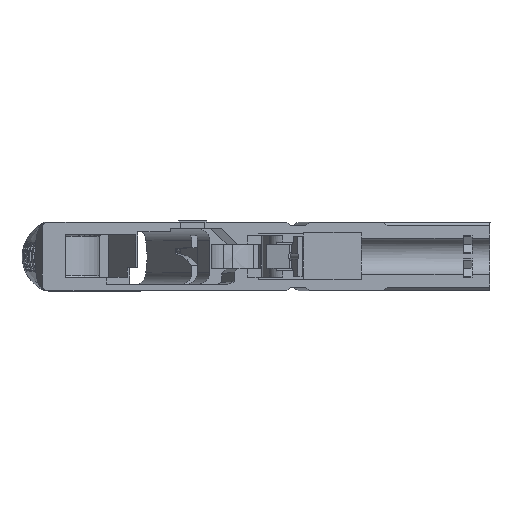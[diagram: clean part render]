
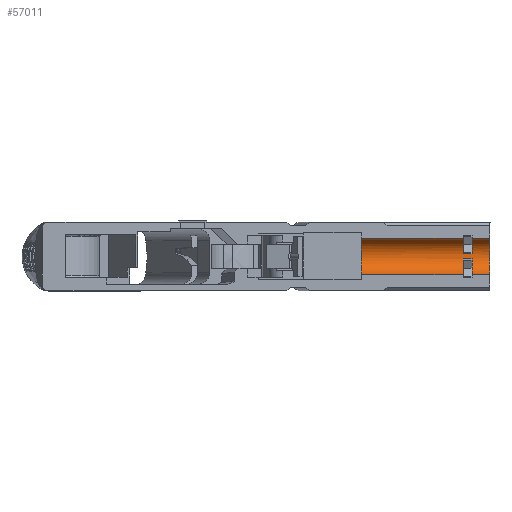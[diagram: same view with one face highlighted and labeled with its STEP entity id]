
A CAD part, top view. The second image highlights one B-rep face of the part: STEP entity #57011.
In plain terms, the highlighted cylindrical face has radius 7.768 mm (diameter 15.535 mm), a partial arc.
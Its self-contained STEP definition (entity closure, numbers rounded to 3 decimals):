
#6073=CYLINDRICAL_SURFACE('',#60469,7.768);
#7816=CIRCLE('',#60417,7.768);
#7819=CIRCLE('',#60444,7.768);
#7824=CIRCLE('',#60450,7.768);
#7827=CIRCLE('',#60465,7.768);
#7828=CIRCLE('',#60467,7.768);
#7829=CIRCLE('',#60470,7.768);
#8081=FACE_OUTER_BOUND('',#11523,.T.);
#11523=EDGE_LOOP('',(#38179,#38180,#38181,#38182,#38183,#38184,#38185,#38186,
#38187,#38188,#38189,#38190,#38191,#38192));
#15564=LINE('',#68849,#19314);
#15572=LINE('',#68868,#19322);
#15574=LINE('',#68871,#19324);
#15575=LINE('',#68873,#19325);
#15576=LINE('',#68876,#19326);
#15577=LINE('',#68877,#19327);
#15578=LINE('',#68879,#19328);
#15579=LINE('',#68880,#19329);
#19314=VECTOR('',#62119,10.);
#19322=VECTOR('',#62139,10.);
#19324=VECTOR('',#62143,10.);
#19325=VECTOR('',#62144,10.);
#19326=VECTOR('',#62147,10.);
#19327=VECTOR('',#62148,10.);
#19328=VECTOR('',#62149,10.);
#19329=VECTOR('',#62150,10.);
#22928=VERTEX_POINT('',#68507);
#22929=VERTEX_POINT('',#68509);
#23008=VERTEX_POINT('',#68746);
#23009=VERTEX_POINT('',#68747);
#23020=VERTEX_POINT('',#68772);
#23021=VERTEX_POINT('',#68773);
#23048=VERTEX_POINT('',#68848);
#23050=VERTEX_POINT('',#68856);
#23051=VERTEX_POINT('',#68857);
#23052=VERTEX_POINT('',#68862);
#23053=VERTEX_POINT('',#68867);
#23054=VERTEX_POINT('',#68872);
#23055=VERTEX_POINT('',#68875);
#23056=VERTEX_POINT('',#68878);
#28901=EDGE_CURVE('',#22928,#22929,#7816,.T.);
#29005=EDGE_CURVE('',#23008,#23009,#7819,.T.);
#29018=EDGE_CURVE('',#23020,#23021,#7824,.T.);
#29056=EDGE_CURVE('',#23048,#23021,#15564,.T.);
#29060=EDGE_CURVE('',#23050,#23051,#7827,.T.);
#29063=EDGE_CURVE('',#23052,#23048,#7828,.T.);
#29066=EDGE_CURVE('',#23052,#23053,#15572,.T.);
#29068=EDGE_CURVE('',#23008,#23050,#15574,.T.);
#29069=EDGE_CURVE('',#23054,#23051,#15575,.T.);
#29070=EDGE_CURVE('',#23053,#23054,#7829,.T.);
#29071=EDGE_CURVE('',#23055,#23020,#15576,.T.);
#29072=EDGE_CURVE('',#22929,#23055,#15577,.T.);
#29073=EDGE_CURVE('',#23056,#22928,#15578,.T.);
#29074=EDGE_CURVE('',#23056,#23009,#15579,.T.);
#38179=ORIENTED_EDGE('',*,*,#29068,.T.);
#38180=ORIENTED_EDGE('',*,*,#29060,.T.);
#38181=ORIENTED_EDGE('',*,*,#29069,.F.);
#38182=ORIENTED_EDGE('',*,*,#29070,.F.);
#38183=ORIENTED_EDGE('',*,*,#29066,.F.);
#38184=ORIENTED_EDGE('',*,*,#29063,.T.);
#38185=ORIENTED_EDGE('',*,*,#29056,.T.);
#38186=ORIENTED_EDGE('',*,*,#29018,.F.);
#38187=ORIENTED_EDGE('',*,*,#29071,.F.);
#38188=ORIENTED_EDGE('',*,*,#29072,.F.);
#38189=ORIENTED_EDGE('',*,*,#28901,.F.);
#38190=ORIENTED_EDGE('',*,*,#29073,.F.);
#38191=ORIENTED_EDGE('',*,*,#29074,.T.);
#38192=ORIENTED_EDGE('',*,*,#29005,.F.);
#57011=ADVANCED_FACE('',(#8081),#6073,.F.);
#60417=AXIS2_PLACEMENT_3D('',#68510,#61888,#61889);
#60444=AXIS2_PLACEMENT_3D('',#68748,#62038,#62039);
#60450=AXIS2_PLACEMENT_3D('',#68774,#62058,#62059);
#60465=AXIS2_PLACEMENT_3D('',#68858,#62127,#62128);
#60467=AXIS2_PLACEMENT_3D('',#68863,#62133,#62134);
#60469=AXIS2_PLACEMENT_3D('',#68870,#62141,#62142);
#60470=AXIS2_PLACEMENT_3D('',#68874,#62145,#62146);
#61888=DIRECTION('center_axis',(-1.,0.,0.));
#61889=DIRECTION('ref_axis',(0.,-1.,0.));
#62038=DIRECTION('center_axis',(1.,0.,0.));
#62039=DIRECTION('ref_axis',(0.,-1.,0.));
#62058=DIRECTION('center_axis',(1.,0.,0.));
#62059=DIRECTION('ref_axis',(0.,-1.,0.));
#62119=DIRECTION('',(1.,0.,0.));
#62127=DIRECTION('center_axis',(1.,0.,0.));
#62128=DIRECTION('ref_axis',(0.,-1.,0.));
#62133=DIRECTION('center_axis',(1.,0.,0.));
#62134=DIRECTION('ref_axis',(0.,-1.,0.));
#62139=DIRECTION('',(-1.,0.,0.));
#62141=DIRECTION('center_axis',(1.,0.,0.));
#62142=DIRECTION('ref_axis',(0.,0.,
-1.));
#62143=DIRECTION('',(-1.,0.,0.));
#62144=DIRECTION('',(1.,0.,0.));
#62145=DIRECTION('center_axis',(1.,0.,0.));
#62146=DIRECTION('ref_axis',(0.,-1.,0.));
#62147=DIRECTION('',(-1.,0.,0.));
#62148=DIRECTION('',(-1.,0.,0.));
#62149=DIRECTION('',(1.,0.,0.));
#62150=DIRECTION('',(-1.,0.,0.));
#68507=CARTESIAN_POINT('',(158.035,34.275,-145.108));
#68509=CARTESIAN_POINT('',(158.035,18.747,-145.108));
#68510=CARTESIAN_POINT('Origin',(158.035,26.511,-145.351));
#68746=CARTESIAN_POINT('',(150.385,27.547,-153.049));
#68747=CARTESIAN_POINT('',(150.385,34.275,-145.108));
#68748=CARTESIAN_POINT('Origin',(150.385,26.511,-145.351));
#68772=CARTESIAN_POINT('',(150.385,18.747,-145.108));
#68773=CARTESIAN_POINT('',(150.385,25.475,-153.049));
#68774=CARTESIAN_POINT('Origin',(150.385,26.511,-145.351));
#68848=CARTESIAN_POINT('',(146.635,25.475,-153.049));
#68849=CARTESIAN_POINT('',(103.12,25.475,-153.049));
#68856=CARTESIAN_POINT('',(146.635,27.547,-153.049));
#68857=CARTESIAN_POINT('',(146.635,34.275,-145.108));
#68858=CARTESIAN_POINT('Origin',(146.635,26.511,-145.351));
#68862=CARTESIAN_POINT('',(146.635,18.747,-145.108));
#68863=CARTESIAN_POINT('Origin',(146.635,26.511,-145.351));
#68867=CARTESIAN_POINT('',(103.12,18.747,-145.108));
#68868=CARTESIAN_POINT('',(103.12,18.747,-145.108));
#68870=CARTESIAN_POINT('Origin',(103.12,26.511,-145.351));
#68871=CARTESIAN_POINT('',(103.12,27.547,-153.049));
#68872=CARTESIAN_POINT('',(103.12,34.275,-145.108));
#68873=CARTESIAN_POINT('',(103.12,34.275,-145.108));
#68874=CARTESIAN_POINT('Origin',(103.12,26.511,-145.351));
#68875=CARTESIAN_POINT('',(152.135,18.747,-145.108));
#68876=CARTESIAN_POINT('',(152.135,18.747,-145.108));
#68877=CARTESIAN_POINT('',(103.12,18.747,-145.108));
#68878=CARTESIAN_POINT('',(152.135,34.275,-145.108));
#68879=CARTESIAN_POINT('',(103.12,34.275,-145.108));
#68880=CARTESIAN_POINT('',(152.135,34.275,-145.108));
